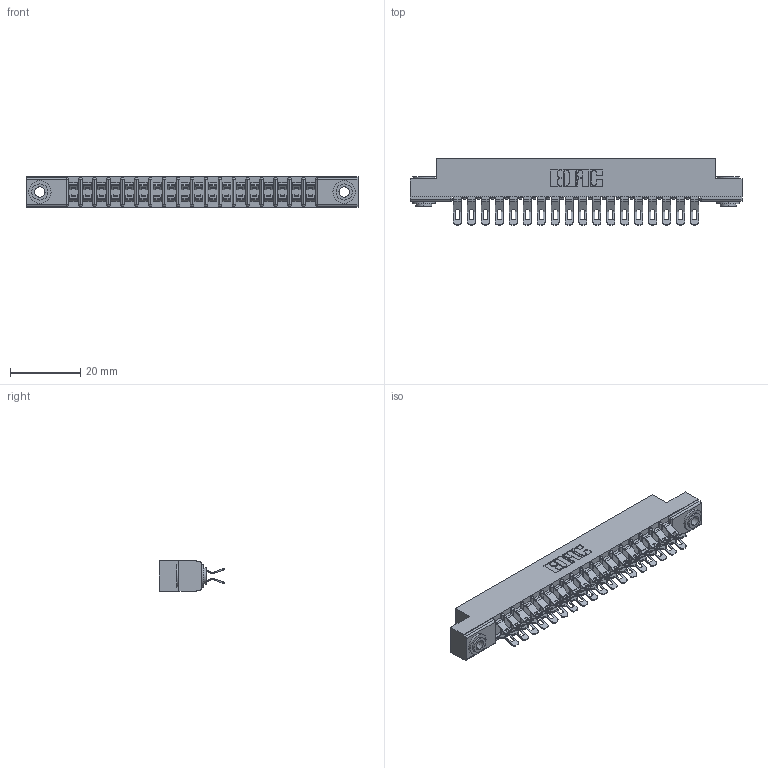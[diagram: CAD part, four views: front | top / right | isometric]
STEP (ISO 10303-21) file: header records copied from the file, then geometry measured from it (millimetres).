
FILE_DESCRIPTION (( 'STEP AP203' ), '1' );
FILE_NAME ('357-036-455-203.STEP', '2020-10-03T17:52:40', ( '' ), ( '' ), 'SwSTEP 2.0', 'SolidWorks 2020', '' );
FILE_SCHEMA (( 'CONFIG_CONTROL_DESIGN' ));
Length unit declared in the file: inch
Products named in the file (4): 307-290-001_555; 345-250-002_345-250-002-102; 307 Part_.156 Dia Mounting Holes; 357-036-455-203
Assembly tree (39 placements, depth 2):
  357-036-455-203
    307 Part_.156 Dia Mounting Holes
    307-290-001_555  x36
    345-250-002_345-250-002-102  x2
Bounding box: 94.34 x 18.75 x 8.71 mm (x, y, z)
Volume: 6279.6 mm3; surface area: 11722.3 mm2
Topology: 39 solids, 39 shells, 2385 faces, 6951 edges, 4530 vertices
Faces by surface type: plane 1318, cylinder 1021, sphere 38, cone 8
Entity records: 20568 total; most frequent: CARTESIAN_POINT 3359, DIRECTION 3322, ORIENTED_EDGE 3320, EDGE_CURVE 1660, LINE 1244, VECTOR 1244, VERTEX_POINT 1076, AXIS2_PLACEMENT_3D 1039
